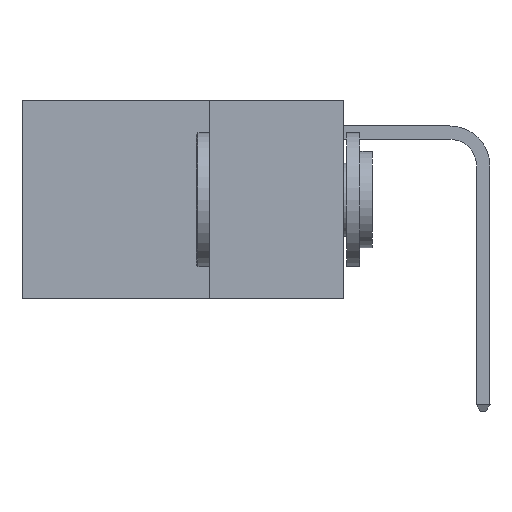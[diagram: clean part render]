
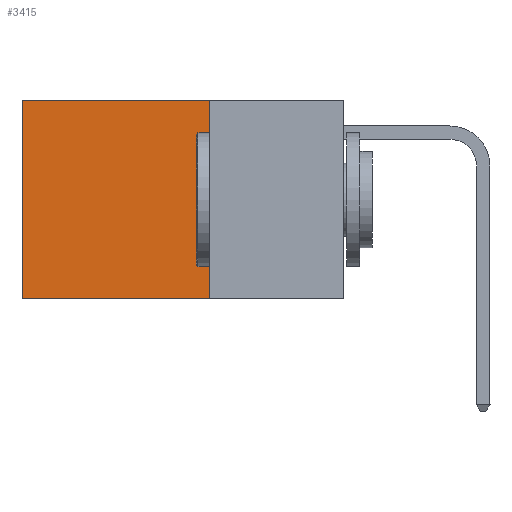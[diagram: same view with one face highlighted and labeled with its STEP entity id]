
A CAD part, left-side view. The second image highlights one B-rep face of the part: STEP entity #3415.
In plain terms, the highlighted planar face has unit normal (-1, 0, 0).
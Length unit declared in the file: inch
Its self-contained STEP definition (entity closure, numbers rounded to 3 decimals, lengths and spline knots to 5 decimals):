
#408 = VERTEX_POINT ( 'NONE', #744 ) ;
#744 = CARTESIAN_POINT ( 'NONE',  ( 0.2625, 0.25, 0. ) ) ;
#837 = CARTESIAN_POINT ( 'NONE',  ( 0.2625, 0.25, -0.37 ) ) ;
#1120 = CARTESIAN_POINT ( 'NONE',  ( 0.2625, 0.6, 0. ) ) ;
#1139 = VECTOR ( 'NONE', #2466, 39.37008 ) ;
#1180 = LINE ( 'NONE', #2514, #1139 ) ;
#1834 = ORIENTED_EDGE ( 'NONE', *, *, #2169, .F. ) ;
#2169 = EDGE_CURVE ( 'NONE', #408, #9201, #2258, .T. ) ;
#2200 = VECTOR ( 'NONE', #8018, 39.37008 ) ;
#2258 = LINE ( 'NONE', #6964, #2200 ) ;
#2466 = DIRECTION ( 'NONE',  ( 0., 0., -1. ) ) ;
#2514 = CARTESIAN_POINT ( 'NONE',  ( 0.2625, 0.6, 0. ) ) ;
#2640 = ORIENTED_EDGE ( 'NONE', *, *, #5037, .T. ) ;
#2826 = DIRECTION ( 'NONE',  ( 0., 0., -1. ) ) ;
#3337 = VERTEX_POINT ( 'NONE', #1120 ) ;
#3351 = VERTEX_POINT ( 'NONE', #7364 ) ;
#3415 = ADVANCED_FACE ( 'NONE', ( #7119 ), #8833, .F. ) ;
#3844 = EDGE_LOOP ( 'NONE', ( #6262, #8680, #1834, #2640 ) ) ;
#4085 = CARTESIAN_POINT ( 'NONE',  ( 0.2625, 0.25, 0. ) ) ;
#4732 = EDGE_CURVE ( 'NONE', #3337, #3351, #1180, .T. ) ;
#5037 = EDGE_CURVE ( 'NONE', #408, #3337, #9223, .T. ) ;
#5441 = DIRECTION ( 'NONE',  ( 1., 0., 0. ) ) ;
#5900 = EDGE_CURVE ( 'NONE', #9201, #3351, #5978, .T. ) ;
#5943 = VECTOR ( 'NONE', #8244, 39.37008 ) ;
#5978 = LINE ( 'NONE', #8280, #5943 ) ;
#6262 = ORIENTED_EDGE ( 'NONE', *, *, #4732, .T. ) ;
#6964 = CARTESIAN_POINT ( 'NONE',  ( 0.2625, 0.25, 0. ) ) ;
#7030 = AXIS2_PLACEMENT_3D ( 'NONE', #4085, #5441, #2826 ) ;
#7119 = FACE_OUTER_BOUND ( 'NONE', #3844, .T. ) ;
#7364 = CARTESIAN_POINT ( 'NONE',  ( 0.2625, 0.6, -0.37 ) ) ;
#7814 = DIRECTION ( 'NONE',  ( 0., 1., 0. ) ) ;
#7863 = CARTESIAN_POINT ( 'NONE',  ( 0.2625, 0.25, 0. ) ) ;
#8018 = DIRECTION ( 'NONE',  ( 0., 0., -1. ) ) ;
#8244 = DIRECTION ( 'NONE',  ( 0., 1., 0. ) ) ;
#8280 = CARTESIAN_POINT ( 'NONE',  ( 0.2625, 0.25, -0.37 ) ) ;
#8680 = ORIENTED_EDGE ( 'NONE', *, *, #5900, .F. ) ;
#8833 = PLANE ( 'NONE',  #7030 ) ;
#9201 = VERTEX_POINT ( 'NONE', #837 ) ;
#9212 = VECTOR ( 'NONE', #7814, 39.37008 ) ;
#9223 = LINE ( 'NONE', #7863, #9212 ) ;
